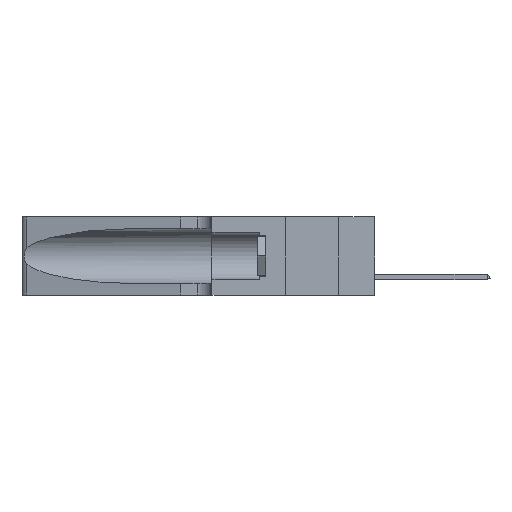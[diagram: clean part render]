
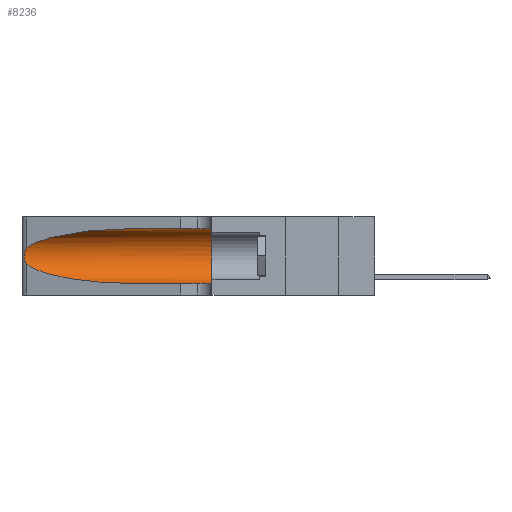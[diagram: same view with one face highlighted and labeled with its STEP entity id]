
A CAD part, left-side view. The second image highlights one B-rep face of the part: STEP entity #8236.
In plain terms, the highlighted cylindrical face has radius 3.308 mm (diameter 6.617 mm), a partial arc.
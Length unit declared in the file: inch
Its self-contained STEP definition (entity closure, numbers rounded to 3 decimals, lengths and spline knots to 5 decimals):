
#848 = EDGE_CURVE ( 'NONE', #41963, #32569, #19770, .T. ) ;
#1998 = CARTESIAN_POINT ( 'NONE',  ( 0.18966, 0.96281, 0.05475 ) ) ;
#2554 = CARTESIAN_POINT ( 'NONE',  ( 0.25639, 1.23184, 0.21858 ) ) ;
#2976 = CARTESIAN_POINT ( 'NONE',  ( 0.26075, 1.23896, 0.178 ) ) ;
#4188 = EDGE_CURVE ( 'NONE', #41963, #6978, #12360, .T. ) ;
#5507 = ORIENTED_EDGE ( 'NONE', *, *, #30448, .F. ) ;
#6978 = VERTEX_POINT ( 'NONE', #14813 ) ;
#7640 = ORIENTED_EDGE ( 'NONE', *, *, #34895, .T. ) ;
#8236 = ADVANCED_FACE ( 'NONE', ( #33461 ), #42403, .F. ) ;
#9256 = VERTEX_POINT ( 'NONE', #33857 ) ;
#9476 = CARTESIAN_POINT ( 'NONE',  ( 0.25856, 1.23593, 0.16098 ) ) ;
#9517 = LINE ( 'NONE', #35594, #38726 ) ;
#9880 = VERTEX_POINT ( 'NONE', #35317 ) ;
#10126 = VERTEX_POINT ( 'NONE', #41600 ) ;
#10380 = DIRECTION ( 'NONE',  ( 0., 0., -1. ) ) ;
#11100 = ORIENTED_EDGE ( 'NONE', *, *, #4188, .T. ) ;
#11977 = CARTESIAN_POINT ( 'NONE',  ( 0.1305, 0.72297, 0.05475 ) ) ;
#12360 =( BOUNDED_CURVE ( )  B_SPLINE_CURVE ( 3, ( #21640, #31681, #35198, #21491 ),
 .UNSPECIFIED., .F., .F. ) 
 B_SPLINE_CURVE_WITH_KNOTS ( ( 4, 4 ),
 ( 1.5708, 2.84003 ),
 .UNSPECIFIED. ) 
 CURVE ( )  GEOMETRIC_REPRESENTATION_ITEM ( )  RATIONAL_B_SPLINE_CURVE ( ( 1., 0.87, 0.87, 1. ) ) 
 REPRESENTATION_ITEM ( '' )  );
#12818 = CARTESIAN_POINT ( 'NONE',  ( 0.25639, 1.23186, 0.15144 ) ) ;
#14376 = EDGE_CURVE ( 'NONE', #6978, #9256, #29416, .T. ) ;
#14813 = CARTESIAN_POINT ( 'NONE',  ( 0.25487, 1.22718, 0.22369 ) ) ;
#15556 = VECTOR ( 'NONE', #41728, 39.37008 ) ;
#16302 = CARTESIAN_POINT ( 'NONE',  ( 0.26018, 1.23835, 0.19895 ) ) ;
#17033 = CARTESIAN_POINT ( 'NONE',  ( 0.25487, 1.22718, 0.14631 ) ) ;
#19565 = CARTESIAN_POINT ( 'NONE',  ( 0.26075, 1.23896, 0.19203 ) ) ;
#19770 = LINE ( 'NONE', #32196, #15556 ) ;
#21491 = CARTESIAN_POINT ( 'NONE',  ( 0.25487, 1.22718, 0.22369 ) ) ;
#21640 = CARTESIAN_POINT ( 'NONE',  ( 0.1305, 0.72297, 0.31525 ) ) ;
#21769 = CIRCLE ( 'NONE', #36665, 0.13025 ) ;
#21771 = DIRECTION ( 'NONE',  ( 0., -1., 0. ) ) ;
#22723 = CARTESIAN_POINT ( 'NONE',  ( 0.25789, 1.23486, 0.15765 ) ) ;
#22855 = CARTESIAN_POINT ( 'NONE',  ( 0.25487, 1.22718, 0.14631 ) ) ;
#22949 = CARTESIAN_POINT ( 'NONE',  ( 0.1305, 0.35, 0.185 ) ) ;
#23759 = DIRECTION ( 'NONE',  ( 0., -1., 0. ) ) ;
#27522 = ORIENTED_EDGE ( 'NONE', *, *, #848, .F. ) ;
#29167 = EDGE_LOOP ( 'NONE', ( #11100, #42999, #30317, #7640, #5507, #27522 ) ) ;
#29309 = CARTESIAN_POINT ( 'NONE',  ( 0.25787, 1.23484, 0.2124 ) ) ;
#29405 = EDGE_CURVE ( 'NONE', #9256, #10126, #35912, .T. ) ;
#29416 = B_SPLINE_CURVE_WITH_KNOTS ( 'NONE', 3,
 ( #39527, #39098, #2554, #29309, #36003, #16302, #19565, #2976, #42775, #9476, #22723, #12818, #42917, #22855 ),
 .UNSPECIFIED., .F., .F.,
 ( 4, 2, 2, 2, 2, 2, 4 ),
 ( 0., 0.00027, 0.00053, 0.00107, 0.0016, 0.00187, 0.00214 ),
 .UNSPECIFIED. ) ;
#30317 = ORIENTED_EDGE ( 'NONE', *, *, #29405, .T. ) ;
#30448 = EDGE_CURVE ( 'NONE', #32569, #9880, #21769, .T. ) ;
#31681 = CARTESIAN_POINT ( 'NONE',  ( 0.18966, 0.96281, 0.31525 ) ) ;
#31804 = CARTESIAN_POINT ( 'NONE',  ( 0.2373, 1.15595, 0.08982 ) ) ;
#32196 = CARTESIAN_POINT ( 'NONE',  ( 0.1305, 1.61858, 0.31525 ) ) ;
#32569 = VERTEX_POINT ( 'NONE', #41968 ) ;
#33461 = FACE_OUTER_BOUND ( 'NONE', #29167, .T. ) ;
#33857 = CARTESIAN_POINT ( 'NONE',  ( 0.25487, 1.22718, 0.14631 ) ) ;
#34895 = EDGE_CURVE ( 'NONE', #10126, #9880, #9517, .T. ) ;
#35198 = CARTESIAN_POINT ( 'NONE',  ( 0.2373, 1.15595, 0.28018 ) ) ;
#35317 = CARTESIAN_POINT ( 'NONE',  ( 0.1305, 0.35, 0.05475 ) ) ;
#35330 = CARTESIAN_POINT ( 'NONE',  ( 0.1305, 0.72297, 0.31525 ) ) ;
#35594 = CARTESIAN_POINT ( 'NONE',  ( 0.1305, 1.61858, 0.05475 ) ) ;
#35912 =( BOUNDED_CURVE ( )  B_SPLINE_CURVE ( 3, ( #17033, #31804, #1998, #11977 ),
 .UNSPECIFIED., .F., .F. ) 
 B_SPLINE_CURVE_WITH_KNOTS ( ( 4, 4 ),
 ( 3.44316, 4.71239 ),
 .UNSPECIFIED. ) 
 CURVE ( )  GEOMETRIC_REPRESENTATION_ITEM ( )  RATIONAL_B_SPLINE_CURVE ( ( 1., 0.87, 0.87, 1. ) ) 
 REPRESENTATION_ITEM ( '' )  );
#36003 = CARTESIAN_POINT ( 'NONE',  ( 0.25854, 1.2359, 0.20912 ) ) ;
#36536 = DIRECTION ( 'NONE',  ( 0., 0., 1. ) ) ;
#36665 = AXIS2_PLACEMENT_3D ( 'NONE', #22949, #39485, #36536 ) ;
#37353 = CARTESIAN_POINT ( 'NONE',  ( 0.1305, 1.61858, 0.185 ) ) ;
#38696 = AXIS2_PLACEMENT_3D ( 'NONE', #37353, #23759, #10380 ) ;
#38726 = VECTOR ( 'NONE', #21771, 39.37008 ) ;
#39098 = CARTESIAN_POINT ( 'NONE',  ( 0.25555, 1.22994, 0.2215 ) ) ;
#39485 = DIRECTION ( 'NONE',  ( 0., 1., 0. ) ) ;
#39527 = CARTESIAN_POINT ( 'NONE',  ( 0.25487, 1.22718, 0.22369 ) ) ;
#41600 = CARTESIAN_POINT ( 'NONE',  ( 0.1305, 0.72297, 0.05475 ) ) ;
#41728 = DIRECTION ( 'NONE',  ( 0., -1., 0. ) ) ;
#41963 = VERTEX_POINT ( 'NONE', #35330 ) ;
#41968 = CARTESIAN_POINT ( 'NONE',  ( 0.1305, 0.35, 0.31525 ) ) ;
#42403 = CYLINDRICAL_SURFACE ( 'NONE', #38696, 0.13025 ) ;
#42775 = CARTESIAN_POINT ( 'NONE',  ( 0.26017, 1.23833, 0.17102 ) ) ;
#42917 = CARTESIAN_POINT ( 'NONE',  ( 0.25555, 1.22993, 0.14849 ) ) ;
#42999 = ORIENTED_EDGE ( 'NONE', *, *, #14376, .T. ) ;
